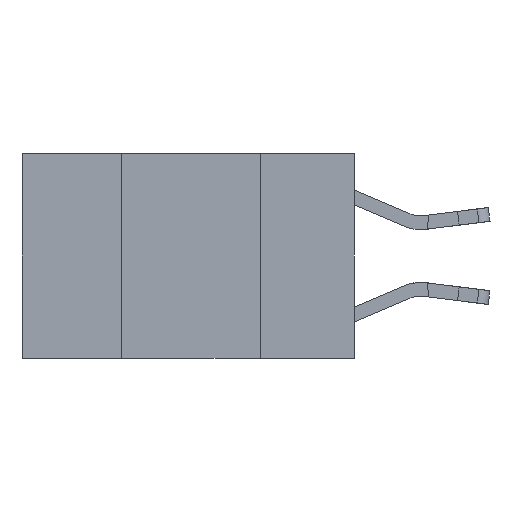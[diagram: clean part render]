
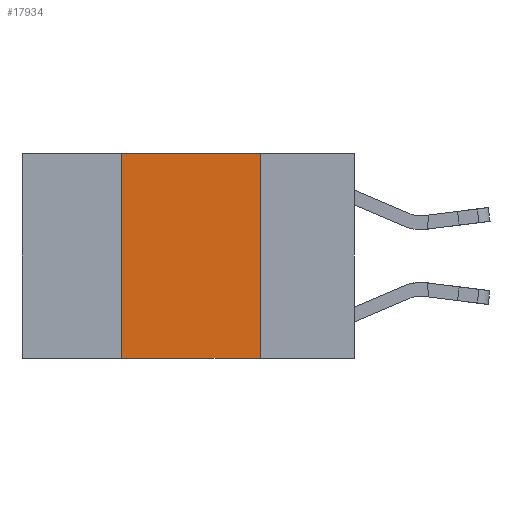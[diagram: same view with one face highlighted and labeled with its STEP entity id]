
A CAD part, left-side view. The second image highlights one B-rep face of the part: STEP entity #17934.
In plain terms, the highlighted planar face has unit normal (-1, 0, 0).
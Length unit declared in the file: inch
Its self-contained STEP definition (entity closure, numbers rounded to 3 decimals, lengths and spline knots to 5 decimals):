
#160 = VERTEX_POINT ( 'NONE', #13326 ) ;
#1902 = LINE ( 'NONE', #2025, #2685 ) ;
#2025 = CARTESIAN_POINT ( 'NONE',  ( 0., 0.17, 0. ) ) ;
#2685 = VECTOR ( 'NONE', #7003, 39.37008 ) ;
#3968 = EDGE_CURVE ( 'NONE', #18915, #12424, #1902, .T. ) ;
#4417 = VECTOR ( 'NONE', #21388, 39.37008 ) ;
#5418 = ORIENTED_EDGE ( 'NONE', *, *, #3968, .F. ) ;
#5463 = CARTESIAN_POINT ( 'NONE',  ( 0., 0.6, 0. ) ) ;
#5682 = DIRECTION ( 'NONE',  ( 0., -1., 0. ) ) ;
#6461 = ORIENTED_EDGE ( 'NONE', *, *, #12118, .F. ) ;
#6669 = AXIS2_PLACEMENT_3D ( 'NONE', #5463, #14599, #7198 ) ;
#7001 = EDGE_CURVE ( 'NONE', #160, #20962, #15469, .T. ) ;
#7003 = DIRECTION ( 'NONE',  ( 0., 0., -1. ) ) ;
#7195 = CARTESIAN_POINT ( 'NONE',  ( 0., 0.6, 0. ) ) ;
#7198 = DIRECTION ( 'NONE',  ( 0., 0., -1. ) ) ;
#7324 = FACE_OUTER_BOUND ( 'NONE', #16428, .T. ) ;
#7663 = LINE ( 'NONE', #7195, #4417 ) ;
#8622 = DIRECTION ( 'NONE',  ( 0., 0., 1. ) ) ;
#9032 = LINE ( 'NONE', #17827, #15761 ) ;
#12118 = EDGE_CURVE ( 'NONE', #20962, #18915, #7663, .T. ) ;
#12185 = ORIENTED_EDGE ( 'NONE', *, *, #7001, .F. ) ;
#12424 = VERTEX_POINT ( 'NONE', #19301 ) ;
#13326 = CARTESIAN_POINT ( 'NONE',  ( 0., 0.42, -0.37 ) ) ;
#13364 = CARTESIAN_POINT ( 'NONE',  ( 0., 0.17, 0. ) ) ;
#14046 = CARTESIAN_POINT ( 'NONE',  ( 0., 0.42, 0. ) ) ;
#14599 = DIRECTION ( 'NONE',  ( 1., 0., 0. ) ) ;
#14814 = VECTOR ( 'NONE', #8622, 39.37008 ) ;
#15229 = EDGE_CURVE ( 'NONE', #160, #12424, #9032, .T. ) ;
#15469 = LINE ( 'NONE', #14046, #14814 ) ;
#15761 = VECTOR ( 'NONE', #5682, 39.37008 ) ;
#15995 = PLANE ( 'NONE',  #6669 ) ;
#16292 = ORIENTED_EDGE ( 'NONE', *, *, #15229, .T. ) ;
#16428 = EDGE_LOOP ( 'NONE', ( #5418, #6461, #12185, #16292 ) ) ;
#17686 = CARTESIAN_POINT ( 'NONE',  ( 0., 0.42, 0. ) ) ;
#17827 = CARTESIAN_POINT ( 'NONE',  ( 0., 0.6, -0.37 ) ) ;
#17934 = ADVANCED_FACE ( 'NONE', ( #7324 ), #15995, .F. ) ;
#18915 = VERTEX_POINT ( 'NONE', #13364 ) ;
#19301 = CARTESIAN_POINT ( 'NONE',  ( 0., 0.17, -0.37 ) ) ;
#20962 = VERTEX_POINT ( 'NONE', #17686 ) ;
#21388 = DIRECTION ( 'NONE',  ( 0., -1., 0. ) ) ;
